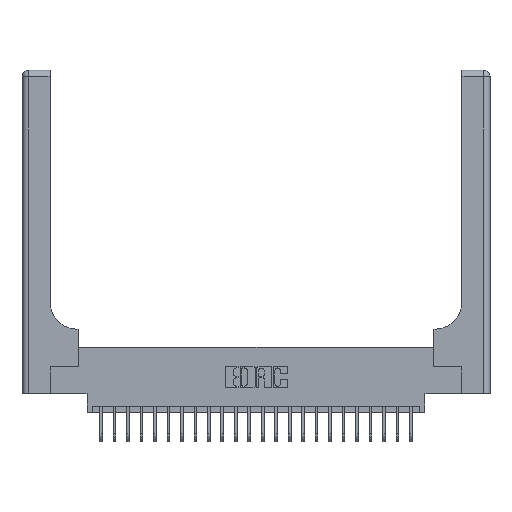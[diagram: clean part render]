
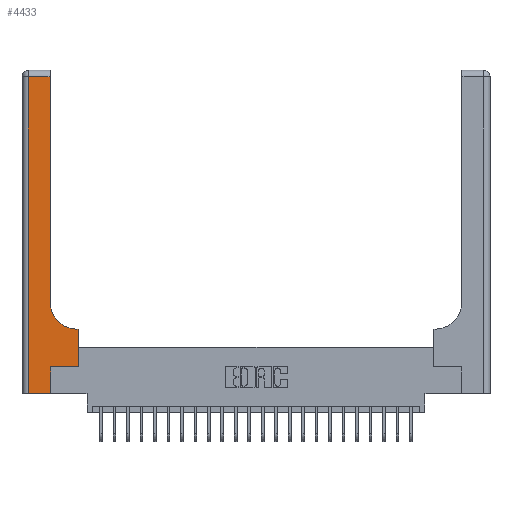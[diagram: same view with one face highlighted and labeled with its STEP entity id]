
A CAD part, top view. The second image highlights one B-rep face of the part: STEP entity #4433.
In plain terms, the highlighted planar face has unit normal (0, 0, 1).
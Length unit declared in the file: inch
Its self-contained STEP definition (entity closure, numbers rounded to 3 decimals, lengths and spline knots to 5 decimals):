
#360 = CARTESIAN_POINT ( 'NONE',  ( 0.265, 0., 0.37 ) ) ;
#950 = ORIENTED_EDGE ( 'NONE', *, *, #17441, .T. ) ;
#986 = EDGE_CURVE ( 'NONE', #11075, #10950, #5448, .T. ) ;
#1209 = CARTESIAN_POINT ( 'NONE',  ( 0.51, 0.85, 0.37 ) ) ;
#1300 = VERTEX_POINT ( 'NONE', #17816 ) ;
#1350 = ORIENTED_EDGE ( 'NONE', *, *, #6255, .T. ) ;
#1669 = ORIENTED_EDGE ( 'NONE', *, *, #986, .T. ) ;
#1960 = CARTESIAN_POINT ( 'NONE',  ( 0.265, 0., 0.37 ) ) ;
#2208 = CARTESIAN_POINT ( 'NONE',  ( 0.26, 2.94, 0.37 ) ) ;
#2651 = DIRECTION ( 'NONE',  ( -1., 0., 0. ) ) ;
#2744 = CARTESIAN_POINT ( 'NONE',  ( 0.06, 3., 0.37 ) ) ;
#2905 = CARTESIAN_POINT ( 'NONE',  ( 0., 3., 0.37 ) ) ;
#3054 = VECTOR ( 'NONE', #22098, 39.37008 ) ;
#3539 = ORIENTED_EDGE ( 'NONE', *, *, #17026, .T. ) ;
#3957 = DIRECTION ( 'NONE',  ( 1., 0., 0. ) ) ;
#4170 = ORIENTED_EDGE ( 'NONE', *, *, #24976, .T. ) ;
#4433 = ADVANCED_FACE ( 'NONE', ( #20724 ), #14969, .F. ) ;
#5147 = VECTOR ( 'NONE', #12657, 39.37008 ) ;
#5342 = DIRECTION ( 'NONE',  ( 1., 0., 0. ) ) ;
#5448 = LINE ( 'NONE', #19613, #6349 ) ;
#5928 = ORIENTED_EDGE ( 'NONE', *, *, #7576, .T. ) ;
#6255 = EDGE_CURVE ( 'NONE', #1300, #6467, #9799, .T. ) ;
#6349 = VECTOR ( 'NONE', #15818, 39.37008 ) ;
#6467 = VERTEX_POINT ( 'NONE', #13739 ) ;
#6545 = DIRECTION ( 'NONE',  ( 0., 1., 0. ) ) ;
#6567 = CARTESIAN_POINT ( 'NONE',  ( 0.06, 2.94, 0.37 ) ) ;
#6758 = DIRECTION ( 'NONE',  ( 0., -1., 0. ) ) ;
#7198 = VECTOR ( 'NONE', #16088, 39.37008 ) ;
#7576 = EDGE_CURVE ( 'NONE', #18688, #19604, #10468, .T. ) ;
#7695 = ORIENTED_EDGE ( 'NONE', *, *, #23022, .T. ) ;
#8175 = CARTESIAN_POINT ( 'NONE',  ( 0.26, 0.6, 0.37 ) ) ;
#8208 = VERTEX_POINT ( 'NONE', #20567 ) ;
#9107 = DIRECTION ( 'NONE',  ( 1., 0., 0. ) ) ;
#9799 = CIRCLE ( 'NONE', #24336, 0.25 ) ;
#9854 = VERTEX_POINT ( 'NONE', #19646 ) ;
#10468 = LINE ( 'NONE', #12525, #5147 ) ;
#10655 = ORIENTED_EDGE ( 'NONE', *, *, #25570, .T. ) ;
#10688 = EDGE_LOOP ( 'NONE', ( #3539, #5928, #7695, #10655, #950, #4170, #1669, #18254, #1350 ) ) ;
#10950 = VERTEX_POINT ( 'NONE', #21367 ) ;
#11075 = VERTEX_POINT ( 'NONE', #17709 ) ;
#11090 = VECTOR ( 'NONE', #6758, 39.37008 ) ;
#11161 = EDGE_CURVE ( 'NONE', #10950, #1300, #19876, .T. ) ;
#11450 = CARTESIAN_POINT ( 'NONE',  ( 0., 0., 0.37 ) ) ;
#11572 = LINE ( 'NONE', #11450, #17621 ) ;
#12458 = VECTOR ( 'NONE', #6545, 39.37008 ) ;
#12525 = CARTESIAN_POINT ( 'NONE',  ( 0., 2.94, 0.37 ) ) ;
#12657 = DIRECTION ( 'NONE',  ( -1., 0., 0. ) ) ;
#12710 = LINE ( 'NONE', #2744, #11090 ) ;
#12744 = CARTESIAN_POINT ( 'NONE',  ( 0.26, 3., 0.37 ) ) ;
#13739 = CARTESIAN_POINT ( 'NONE',  ( 0.26, 0.85, 0.37 ) ) ;
#14148 = LINE ( 'NONE', #1960, #3054 ) ;
#14969 = PLANE ( 'NONE',  #17691 ) ;
#15818 = DIRECTION ( 'NONE',  ( 0., 1., 0. ) ) ;
#16088 = DIRECTION ( 'NONE',  ( -1., 0., 0. ) ) ;
#17026 = EDGE_CURVE ( 'NONE', #6467, #18688, #18988, .T. ) ;
#17416 = DIRECTION ( 'NONE',  ( 0., 0., -1. ) ) ;
#17441 = EDGE_CURVE ( 'NONE', #20771, #9854, #14148, .T. ) ;
#17621 = VECTOR ( 'NONE', #5342, 39.37008 ) ;
#17691 = AXIS2_PLACEMENT_3D ( 'NONE', #2905, #24364, #2651 ) ;
#17709 = CARTESIAN_POINT ( 'NONE',  ( 0.528, 0.25, 0.37 ) ) ;
#17816 = CARTESIAN_POINT ( 'NONE',  ( 0.51, 0.6, 0.37 ) ) ;
#18254 = ORIENTED_EDGE ( 'NONE', *, *, #11161, .T. ) ;
#18688 = VERTEX_POINT ( 'NONE', #2208 ) ;
#18988 = LINE ( 'NONE', #12744, #12458 ) ;
#19604 = VERTEX_POINT ( 'NONE', #6567 ) ;
#19613 = CARTESIAN_POINT ( 'NONE',  ( 0.528, 0.25, 0.37 ) ) ;
#19646 = CARTESIAN_POINT ( 'NONE',  ( 0.265, 0.25, 0.37 ) ) ;
#19876 = LINE ( 'NONE', #8175, #7198 ) ;
#20096 = VECTOR ( 'NONE', #3957, 39.37008 ) ;
#20567 = CARTESIAN_POINT ( 'NONE',  ( 0.06, 0., 0.37 ) ) ;
#20724 = FACE_OUTER_BOUND ( 'NONE', #10688, .T. ) ;
#20771 = VERTEX_POINT ( 'NONE', #360 ) ;
#21367 = CARTESIAN_POINT ( 'NONE',  ( 0.528, 0.6, 0.37 ) ) ;
#21787 = CARTESIAN_POINT ( 'NONE',  ( 0.265, 0.25, 0.37 ) ) ;
#22098 = DIRECTION ( 'NONE',  ( 0., 1., 0. ) ) ;
#23022 = EDGE_CURVE ( 'NONE', #19604, #8208, #12710, .T. ) ;
#23231 = LINE ( 'NONE', #21787, #20096 ) ;
#24336 = AXIS2_PLACEMENT_3D ( 'NONE', #1209, #17416, #9107 ) ;
#24364 = DIRECTION ( 'NONE',  ( 0., 0., -1. ) ) ;
#24976 = EDGE_CURVE ( 'NONE', #9854, #11075, #23231, .T. ) ;
#25570 = EDGE_CURVE ( 'NONE', #8208, #20771, #11572, .T. ) ;
